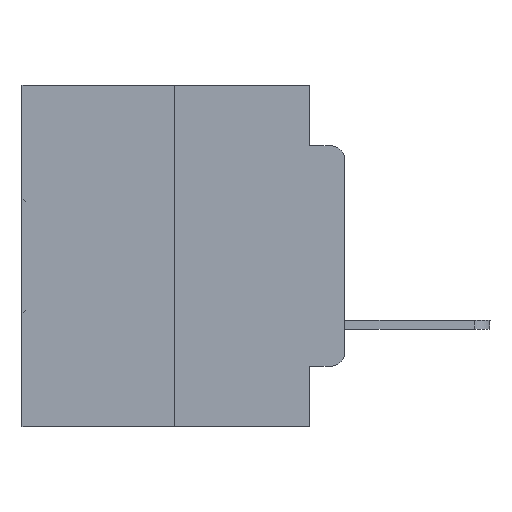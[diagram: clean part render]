
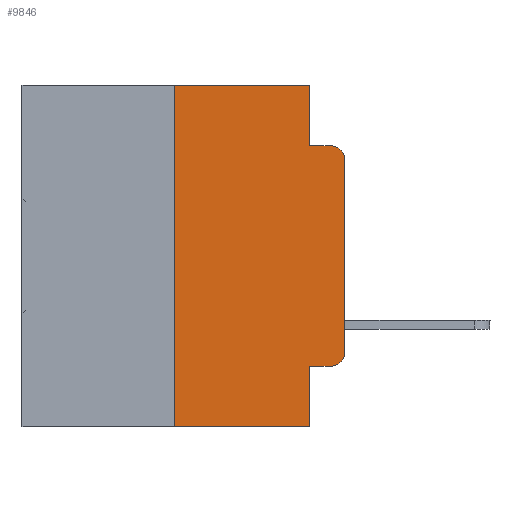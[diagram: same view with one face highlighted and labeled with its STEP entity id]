
A CAD part, left-side view. The second image highlights one B-rep face of the part: STEP entity #9846.
In plain terms, the highlighted planar face has unit normal (-1, 0, 0).
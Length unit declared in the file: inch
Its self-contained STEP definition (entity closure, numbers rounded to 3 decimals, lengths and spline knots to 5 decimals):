
#41 = AXIS2_PLACEMENT_3D ( 'NONE', #21386, #1685, #1475 ) ;
#504 = DIRECTION ( 'NONE',  ( 0., 0., 1. ) ) ;
#522 = VECTOR ( 'NONE', #1225, 39.37008 ) ;
#1225 = DIRECTION ( 'NONE',  ( 0., 0., -1. ) ) ;
#1475 = DIRECTION ( 'NONE',  ( 0., 0., -1. ) ) ;
#1575 = CARTESIAN_POINT ( 'NONE',  ( 0., 0.473, -0.5 ) ) ;
#1616 = EDGE_CURVE ( 'NONE', #2975, #14198, #19688, .T. ) ;
#1685 = DIRECTION ( 'NONE',  ( 1., 0., 0. ) ) ;
#2041 = DIRECTION ( 'NONE',  ( 0., -1., 0. ) ) ;
#2165 = ORIENTED_EDGE ( 'NONE', *, *, #1616, .F. ) ;
#2665 = EDGE_CURVE ( 'NONE', #8073, #5012, #17299, .T. ) ;
#2975 = VERTEX_POINT ( 'NONE', #31124 ) ;
#3272 = FACE_OUTER_BOUND ( 'NONE', #16109, .T. ) ;
#3437 = CARTESIAN_POINT ( 'NONE',  ( 0., 0.051, 0. ) ) ;
#4388 = LINE ( 'NONE', #9177, #29493 ) ;
#5012 = VERTEX_POINT ( 'NONE', #22723 ) ;
#5100 = VERTEX_POINT ( 'NONE', #30389 ) ;
#5737 = EDGE_CURVE ( 'NONE', #5012, #28586, #18192, .T. ) ;
#6506 = DIRECTION ( 'NONE',  ( 0., -1., 0. ) ) ;
#6630 = DIRECTION ( 'NONE',  ( 0., 0., -1. ) ) ;
#6633 = ORIENTED_EDGE ( 'NONE', *, *, #13097, .F. ) ;
#6851 = CARTESIAN_POINT ( 'NONE',  ( 0., 0.02, -0.1085 ) ) ;
#7144 = VERTEX_POINT ( 'NONE', #23646 ) ;
#7705 = ORIENTED_EDGE ( 'NONE', *, *, #2665, .T. ) ;
#7912 = CARTESIAN_POINT ( 'NONE',  ( 0., 0., 0. ) ) ;
#8068 = EDGE_CURVE ( 'NONE', #24295, #22081, #15694, .T. ) ;
#8073 = VERTEX_POINT ( 'NONE', #26516 ) ;
#9108 = CARTESIAN_POINT ( 'NONE',  ( 0., 0., -0.1085 ) ) ;
#9177 = CARTESIAN_POINT ( 'NONE',  ( 0., 0.051, -0.4115 ) ) ;
#9838 = EDGE_CURVE ( 'NONE', #7144, #11590, #12183, .T. ) ;
#9846 = ADVANCED_FACE ( 'NONE', ( #3272 ), #23985, .F. ) ;
#10454 = EDGE_CURVE ( 'NONE', #28586, #22081, #29078, .T. ) ;
#10770 = VECTOR ( 'NONE', #504, 39.37008 ) ;
#10946 = EDGE_CURVE ( 'NONE', #14198, #24295, #18647, .T. ) ;
#11322 = VECTOR ( 'NONE', #13361, 39.37008 ) ;
#11486 = CARTESIAN_POINT ( 'NONE',  ( 0., 0.051, -0.5 ) ) ;
#11590 = VERTEX_POINT ( 'NONE', #11486 ) ;
#12183 = LINE ( 'NONE', #1575, #22586 ) ;
#12748 = DIRECTION ( 'NONE',  ( 0., 0., -1. ) ) ;
#12834 = VECTOR ( 'NONE', #15415, 39.37008 ) ;
#13097 = EDGE_CURVE ( 'NONE', #7144, #2975, #27747, .T. ) ;
#13361 = DIRECTION ( 'NONE',  ( 0., 0., -1. ) ) ;
#13766 = CARTESIAN_POINT ( 'NONE',  ( 0., 0.051, -0.0885 ) ) ;
#14119 = CARTESIAN_POINT ( 'NONE',  ( 0., 0.051, 0. ) ) ;
#14198 = VERTEX_POINT ( 'NONE', #14119 ) ;
#14330 = ORIENTED_EDGE ( 'NONE', *, *, #26977, .F. ) ;
#15411 = DIRECTION ( 'NONE',  ( -1., 0., 0. ) ) ;
#15415 = DIRECTION ( 'NONE',  ( 0., 0., 1. ) ) ;
#15684 = ORIENTED_EDGE ( 'NONE', *, *, #9838, .T. ) ;
#15694 = LINE ( 'NONE', #18864, #29986 ) ;
#15999 = ORIENTED_EDGE ( 'NONE', *, *, #5737, .T. ) ;
#16036 = ORIENTED_EDGE ( 'NONE', *, *, #8068, .F. ) ;
#16109 = EDGE_LOOP ( 'NONE', ( #15999, #18749, #16036, #25967, #2165, #6633, #15684, #14330, #17793, #7705 ) ) ;
#17299 = CIRCLE ( 'NONE', #23631, 0.02 ) ;
#17793 = ORIENTED_EDGE ( 'NONE', *, *, #19467, .T. ) ;
#18192 = LINE ( 'NONE', #7912, #12834 ) ;
#18647 = LINE ( 'NONE', #3437, #11322 ) ;
#18749 = ORIENTED_EDGE ( 'NONE', *, *, #10454, .T. ) ;
#18864 = CARTESIAN_POINT ( 'NONE',  ( 0., 0.051, -0.0885 ) ) ;
#19467 = EDGE_CURVE ( 'NONE', #5100, #8073, #4388, .T. ) ;
#19688 = LINE ( 'NONE', #23915, #22004 ) ;
#20017 = CARTESIAN_POINT ( 'NONE',  ( 0., 0.25, 0. ) ) ;
#21386 = CARTESIAN_POINT ( 'NONE',  ( 0., 0.473, 0. ) ) ;
#22004 = VECTOR ( 'NONE', #29223, 39.37008 ) ;
#22081 = VERTEX_POINT ( 'NONE', #24626 ) ;
#22586 = VECTOR ( 'NONE', #28840, 39.37008 ) ;
#22723 = CARTESIAN_POINT ( 'NONE',  ( 0., 0., -0.3915 ) ) ;
#23302 = CARTESIAN_POINT ( 'NONE',  ( 0., 0.051, 0. ) ) ;
#23631 = AXIS2_PLACEMENT_3D ( 'NONE', #27503, #15411, #12748 ) ;
#23646 = CARTESIAN_POINT ( 'NONE',  ( 0., 0.25, -0.5 ) ) ;
#23915 = CARTESIAN_POINT ( 'NONE',  ( 0., 0.473, 0. ) ) ;
#23985 = PLANE ( 'NONE',  #41 ) ;
#24208 = AXIS2_PLACEMENT_3D ( 'NONE', #6851, #31435, #6630 ) ;
#24295 = VERTEX_POINT ( 'NONE', #13766 ) ;
#24626 = CARTESIAN_POINT ( 'NONE',  ( 0., 0.02, -0.0885 ) ) ;
#25967 = ORIENTED_EDGE ( 'NONE', *, *, #10946, .F. ) ;
#26516 = CARTESIAN_POINT ( 'NONE',  ( 0., 0.02, -0.4115 ) ) ;
#26977 = EDGE_CURVE ( 'NONE', #5100, #11590, #31024, .T. ) ;
#27503 = CARTESIAN_POINT ( 'NONE',  ( 0., 0.02, -0.3915 ) ) ;
#27747 = LINE ( 'NONE', #20017, #10770 ) ;
#28586 = VERTEX_POINT ( 'NONE', #9108 ) ;
#28840 = DIRECTION ( 'NONE',  ( 0., -1., 0. ) ) ;
#29078 = CIRCLE ( 'NONE', #24208, 0.02 ) ;
#29223 = DIRECTION ( 'NONE',  ( 0., -1., 0. ) ) ;
#29493 = VECTOR ( 'NONE', #2041, 39.37008 ) ;
#29986 = VECTOR ( 'NONE', #6506, 39.37008 ) ;
#30389 = CARTESIAN_POINT ( 'NONE',  ( 0., 0.051, -0.4115 ) ) ;
#31024 = LINE ( 'NONE', #23302, #522 ) ;
#31124 = CARTESIAN_POINT ( 'NONE',  ( 0., 0.25, 0. ) ) ;
#31435 = DIRECTION ( 'NONE',  ( -1., 0., 0. ) ) ;
